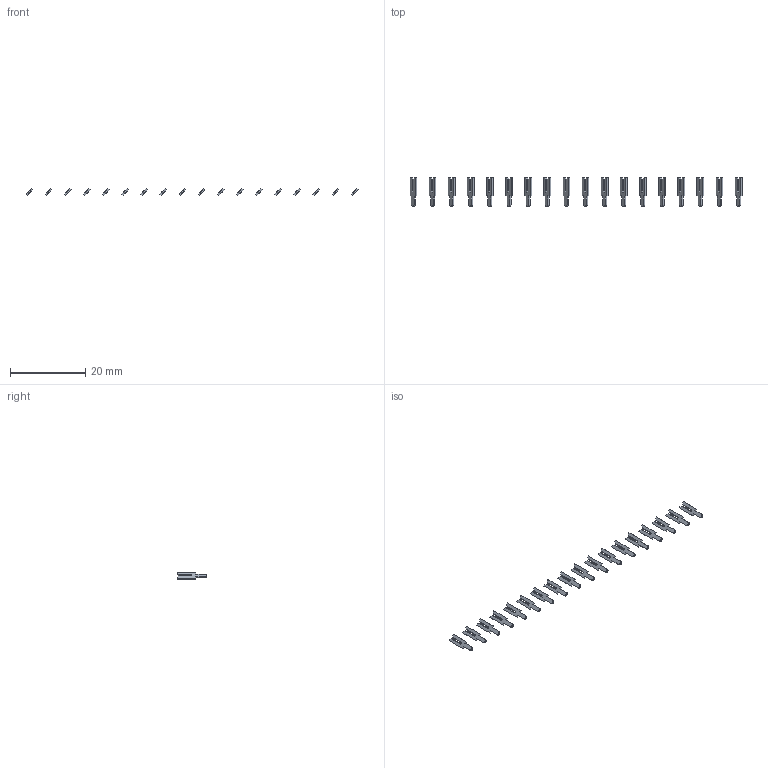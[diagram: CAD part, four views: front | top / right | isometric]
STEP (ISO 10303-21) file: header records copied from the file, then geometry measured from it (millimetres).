
FILE_DESCRIPTION (( 'STEP AP203' ), '1' );
FILE_NAME ('106-018-253-200.STEP', '2020-04-16T18:41:54', ( '' ), ( '' ), 'SwSTEP 2.0', 'SolidWorks 2016', '' );
FILE_SCHEMA (( 'CONFIG_CONTROL_DESIGN' ));
Length unit declared in the file: inch
Products named in the file (2): 106-018-253-200; 100-290-001_100-290-253
Assembly tree (18 placements, depth 2):
  106-018-253-200
    100-290-001_100-290-253  x18
Bounding box: 88.16 x 7.62 x 1.8 mm (x, y, z)
Volume: 99.3 mm3; surface area: 619.3 mm2
Topology: 18 solids, 18 shells, 360 faces, 972 edges, 648 vertices
Faces by surface type: plane 342, cylinder 18
Entity records: 1364 total; most frequent: DIRECTION 138, CARTESIAN_POINT 131, ORIENTED_EDGE 108, EDGE_CURVE 54, LINE 52, VECTOR 52, DATE_AND_TIME 46, CALENDAR_DATE 46
